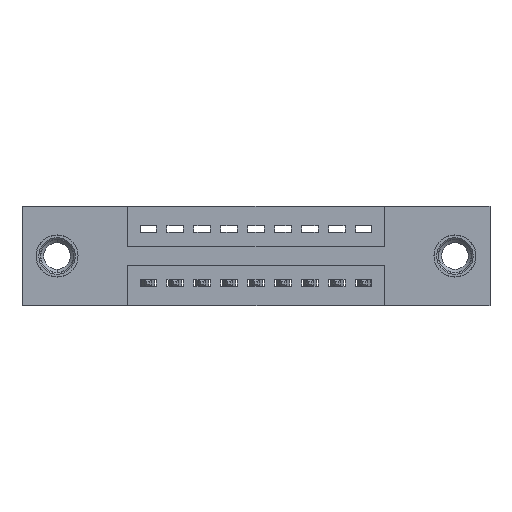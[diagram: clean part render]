
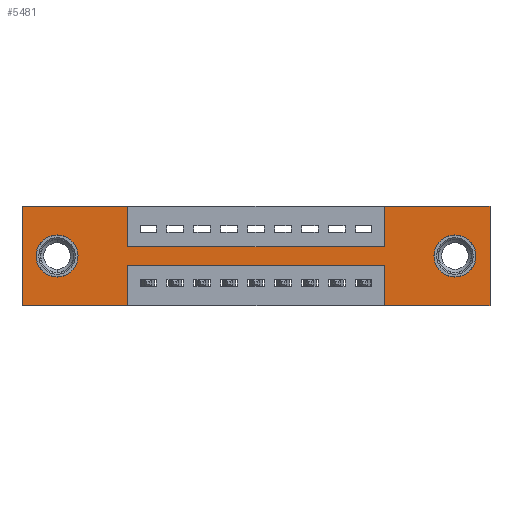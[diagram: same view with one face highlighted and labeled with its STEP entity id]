
A CAD part, front view. The second image highlights one B-rep face of the part: STEP entity #5481.
In plain terms, the highlighted planar face has unit normal (0, -1, 0).
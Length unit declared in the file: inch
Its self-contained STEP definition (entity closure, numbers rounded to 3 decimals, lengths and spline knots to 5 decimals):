
#288 = VECTOR ( 'NONE', #3596, 39.37008 ) ;
#349 = CARTESIAN_POINT ( 'NONE',  ( 1.605, 0., -0.185 ) ) ;
#390 = CIRCLE ( 'NONE', #5759, 0.078 ) ;
#465 = VERTEX_POINT ( 'NONE', #4016 ) ;
#560 = VERTEX_POINT ( 'NONE', #9679 ) ;
#705 = DIRECTION ( 'NONE',  ( 0., 0., -1. ) ) ;
#1059 = CARTESIAN_POINT ( 'NONE',  ( 0., 0., -0.37 ) ) ;
#1062 = CARTESIAN_POINT ( 'NONE',  ( 1.605, 0., -0.263 ) ) ;
#1087 = DIRECTION ( 'NONE',  ( 0., 1., 0. ) ) ;
#1147 = VECTOR ( 'NONE', #7812, 39.37008 ) ;
#1221 = VERTEX_POINT ( 'NONE', #8726 ) ;
#1239 = LINE ( 'NONE', #10455, #8635 ) ;
#1318 = FACE_BOUND ( 'NONE', #9086, .T. ) ;
#1320 = EDGE_CURVE ( 'NONE', #8238, #1763, #4493, .T. ) ;
#1367 = ORIENTED_EDGE ( 'NONE', *, *, #8337, .T. ) ;
#1380 = CARTESIAN_POINT ( 'NONE',  ( 1.3425, 0., -0.37 ) ) ;
#1414 = DIRECTION ( 'NONE',  ( 0., 0., -1. ) ) ;
#1483 = CARTESIAN_POINT ( 'NONE',  ( 0.3925, 0., 0. ) ) ;
#1697 = LINE ( 'NONE', #1380, #11542 ) ;
#1713 = CARTESIAN_POINT ( 'NONE',  ( 0.3925, 0., -0.22 ) ) ;
#1763 = VERTEX_POINT ( 'NONE', #12327 ) ;
#2135 = CARTESIAN_POINT ( 'NONE',  ( 0., 0., -0.37 ) ) ;
#2170 = CARTESIAN_POINT ( 'NONE',  ( 0., 0., -0.37 ) ) ;
#2295 = VERTEX_POINT ( 'NONE', #7875 ) ;
#2490 = EDGE_CURVE ( 'NONE', #6309, #8238, #1239, .T. ) ;
#2916 = LINE ( 'NONE', #3242, #7732 ) ;
#2983 = LINE ( 'NONE', #4534, #288 ) ;
#3011 = CARTESIAN_POINT ( 'NONE',  ( 0.3925, 0., -0.22 ) ) ;
#3021 = VERTEX_POINT ( 'NONE', #3043 ) ;
#3029 = VECTOR ( 'NONE', #6966, 39.37008 ) ;
#3043 = CARTESIAN_POINT ( 'NONE',  ( 0.13, 0., -0.263 ) ) ;
#3197 = VERTEX_POINT ( 'NONE', #1062 ) ;
#3242 = CARTESIAN_POINT ( 'NONE',  ( 0.3925, 0., -0.37 ) ) ;
#3250 = EDGE_CURVE ( 'NONE', #11455, #3021, #390, .T. ) ;
#3339 = CARTESIAN_POINT ( 'NONE',  ( 0.13, 0., -0.107 ) ) ;
#3596 = DIRECTION ( 'NONE',  ( 1., 0., 0. ) ) ;
#3654 = LINE ( 'NONE', #2135, #3029 ) ;
#3747 = LINE ( 'NONE', #6750, #8816 ) ;
#3754 = DIRECTION ( 'NONE',  ( 0., 1., 0. ) ) ;
#3777 = LINE ( 'NONE', #10648, #1147 ) ;
#3824 = DIRECTION ( 'NONE',  ( 0., 0., 1. ) ) ;
#3928 = VERTEX_POINT ( 'NONE', #6061 ) ;
#4016 = CARTESIAN_POINT ( 'NONE',  ( 0.3925, 0., -0.37 ) ) ;
#4255 = ORIENTED_EDGE ( 'NONE', *, *, #10203, .F. ) ;
#4257 = FACE_OUTER_BOUND ( 'NONE', #5708, .T. ) ;
#4493 = LINE ( 'NONE', #7409, #9558 ) ;
#4534 = CARTESIAN_POINT ( 'NONE',  ( 0.3925, 0., -0.15 ) ) ;
#4788 = ORIENTED_EDGE ( 'NONE', *, *, #9786, .T. ) ;
#5016 = DIRECTION ( 'NONE',  ( -1., 0., 0. ) ) ;
#5049 = CARTESIAN_POINT ( 'NONE',  ( 1.3425, 0., -0.22 ) ) ;
#5087 = EDGE_CURVE ( 'NONE', #465, #7644, #3654, .T. ) ;
#5103 = ORIENTED_EDGE ( 'NONE', *, *, #3250, .T. ) ;
#5397 = VECTOR ( 'NONE', #9446, 39.37008 ) ;
#5481 = ADVANCED_FACE ( 'NONE', ( #1318, #6528, #4257 ), #11275, .T. ) ;
#5586 = CIRCLE ( 'NONE', #11164, 0.078 ) ;
#5625 = DIRECTION ( 'NONE',  ( 0., 1., 0. ) ) ;
#5661 = CARTESIAN_POINT ( 'NONE',  ( 0., 0., -0.37 ) ) ;
#5683 = EDGE_CURVE ( 'NONE', #1763, #8829, #3777, .T. ) ;
#5708 = EDGE_LOOP ( 'NONE', ( #4255, #5980, #7627, #7581, #7399, #7213, #6256, #11023, #7398, #10986, #7903, #9835 ) ) ;
#5759 = AXIS2_PLACEMENT_3D ( 'NONE', #6928, #1087, #7863 ) ;
#5768 = ORIENTED_EDGE ( 'NONE', *, *, #7476, .T. ) ;
#5845 = CIRCLE ( 'NONE', #7458, 0.078 ) ;
#5980 = ORIENTED_EDGE ( 'NONE', *, *, #6327, .F. ) ;
#6061 = CARTESIAN_POINT ( 'NONE',  ( 1.3425, 0., -0.37 ) ) ;
#6256 = ORIENTED_EDGE ( 'NONE', *, *, #2490, .F. ) ;
#6309 = VERTEX_POINT ( 'NONE', #12356 ) ;
#6327 = EDGE_CURVE ( 'NONE', #9417, #6745, #9594, .T. ) ;
#6496 = LINE ( 'NONE', #1483, #8671 ) ;
#6528 = FACE_BOUND ( 'NONE', #11121, .T. ) ;
#6612 = DIRECTION ( 'NONE',  ( 0., -1., 0. ) ) ;
#6745 = VERTEX_POINT ( 'NONE', #1713 ) ;
#6750 = CARTESIAN_POINT ( 'NONE',  ( 0., 0., 0. ) ) ;
#6909 = CIRCLE ( 'NONE', #11816, 0.078 ) ;
#6928 = CARTESIAN_POINT ( 'NONE',  ( 0.13, 0., -0.185 ) ) ;
#6966 = DIRECTION ( 'NONE',  ( -1., 0., 0. ) ) ;
#7110 = DIRECTION ( 'NONE',  ( 0., 0., -1. ) ) ;
#7213 = ORIENTED_EDGE ( 'NONE', *, *, #1320, .F. ) ;
#7218 = DIRECTION ( 'NONE',  ( 0., 1., 0. ) ) ;
#7274 = EDGE_CURVE ( 'NONE', #9657, #560, #6496, .T. ) ;
#7348 = EDGE_CURVE ( 'NONE', #560, #6309, #2983, .T. ) ;
#7398 = ORIENTED_EDGE ( 'NONE', *, *, #7274, .F. ) ;
#7399 = ORIENTED_EDGE ( 'NONE', *, *, #5683, .F. ) ;
#7409 = CARTESIAN_POINT ( 'NONE',  ( 0., 0., 0. ) ) ;
#7458 = AXIS2_PLACEMENT_3D ( 'NONE', #11235, #5625, #12114 ) ;
#7476 = EDGE_CURVE ( 'NONE', #3197, #2295, #6909, .T. ) ;
#7543 = EDGE_CURVE ( 'NONE', #7644, #1221, #3747, .T. ) ;
#7581 = ORIENTED_EDGE ( 'NONE', *, *, #8830, .F. ) ;
#7627 = ORIENTED_EDGE ( 'NONE', *, *, #10281, .F. ) ;
#7644 = VERTEX_POINT ( 'NONE', #1059 ) ;
#7732 = VECTOR ( 'NONE', #7110, 39.37008 ) ;
#7812 = DIRECTION ( 'NONE',  ( 0., 0., -1. ) ) ;
#7863 = DIRECTION ( 'NONE',  ( 0., 0., 1. ) ) ;
#7875 = CARTESIAN_POINT ( 'NONE',  ( 1.605, 0., -0.107 ) ) ;
#7903 = ORIENTED_EDGE ( 'NONE', *, *, #7543, .F. ) ;
#8175 = LINE ( 'NONE', #12166, #5397 ) ;
#8238 = VERTEX_POINT ( 'NONE', #11754 ) ;
#8337 = EDGE_CURVE ( 'NONE', #2295, #3197, #5586, .T. ) ;
#8489 = VECTOR ( 'NONE', #10800, 39.37008 ) ;
#8514 = AXIS2_PLACEMENT_3D ( 'NONE', #5661, #6612, #705 ) ;
#8635 = VECTOR ( 'NONE', #10015, 39.37008 ) ;
#8671 = VECTOR ( 'NONE', #11081, 39.37008 ) ;
#8726 = CARTESIAN_POINT ( 'NONE',  ( 0., 0., 0. ) ) ;
#8816 = VECTOR ( 'NONE', #3824, 39.37008 ) ;
#8829 = VERTEX_POINT ( 'NONE', #11661 ) ;
#8830 = EDGE_CURVE ( 'NONE', #8829, #3928, #11004, .T. ) ;
#8981 = VECTOR ( 'NONE', #5016, 39.37008 ) ;
#9086 = EDGE_LOOP ( 'NONE', ( #1367, #5768 ) ) ;
#9324 = EDGE_CURVE ( 'NONE', #1221, #9657, #8175, .T. ) ;
#9417 = VERTEX_POINT ( 'NONE', #5049 ) ;
#9446 = DIRECTION ( 'NONE',  ( 1., 0., 0. ) ) ;
#9471 = CARTESIAN_POINT ( 'NONE',  ( 1.605, 0., -0.185 ) ) ;
#9558 = VECTOR ( 'NONE', #11094, 39.37008 ) ;
#9594 = LINE ( 'NONE', #3011, #8981 ) ;
#9657 = VERTEX_POINT ( 'NONE', #11042 ) ;
#9679 = CARTESIAN_POINT ( 'NONE',  ( 0.3925, 0., -0.15 ) ) ;
#9786 = EDGE_CURVE ( 'NONE', #3021, #11455, #5845, .T. ) ;
#9835 = ORIENTED_EDGE ( 'NONE', *, *, #5087, .F. ) ;
#10015 = DIRECTION ( 'NONE',  ( 0., 0., 1. ) ) ;
#10203 = EDGE_CURVE ( 'NONE', #6745, #465, #2916, .T. ) ;
#10281 = EDGE_CURVE ( 'NONE', #3928, #9417, #1697, .T. ) ;
#10433 = DIRECTION ( 'NONE',  ( 0., 0., -1. ) ) ;
#10455 = CARTESIAN_POINT ( 'NONE',  ( 1.3425, 0., 0. ) ) ;
#10648 = CARTESIAN_POINT ( 'NONE',  ( 1.735, 0., 0. ) ) ;
#10800 = DIRECTION ( 'NONE',  ( -1., 0., 0. ) ) ;
#10986 = ORIENTED_EDGE ( 'NONE', *, *, #9324, .F. ) ;
#11004 = LINE ( 'NONE', #2170, #8489 ) ;
#11023 = ORIENTED_EDGE ( 'NONE', *, *, #7348, .F. ) ;
#11042 = CARTESIAN_POINT ( 'NONE',  ( 0.3925, 0., 0. ) ) ;
#11081 = DIRECTION ( 'NONE',  ( 0., 0., -1. ) ) ;
#11094 = DIRECTION ( 'NONE',  ( 1., 0., 0. ) ) ;
#11121 = EDGE_LOOP ( 'NONE', ( #5103, #4788 ) ) ;
#11164 = AXIS2_PLACEMENT_3D ( 'NONE', #349, #7218, #1414 ) ;
#11235 = CARTESIAN_POINT ( 'NONE',  ( 0.13, 0., -0.185 ) ) ;
#11275 = PLANE ( 'NONE',  #8514 ) ;
#11455 = VERTEX_POINT ( 'NONE', #3339 ) ;
#11542 = VECTOR ( 'NONE', #11883, 39.37008 ) ;
#11661 = CARTESIAN_POINT ( 'NONE',  ( 1.735, 0., -0.37 ) ) ;
#11754 = CARTESIAN_POINT ( 'NONE',  ( 1.3425, 0., 0. ) ) ;
#11816 = AXIS2_PLACEMENT_3D ( 'NONE', #9471, #3754, #10433 ) ;
#11883 = DIRECTION ( 'NONE',  ( 0., 0., 1. ) ) ;
#12114 = DIRECTION ( 'NONE',  ( 0., 0., 1. ) ) ;
#12166 = CARTESIAN_POINT ( 'NONE',  ( 0., 0., 0. ) ) ;
#12327 = CARTESIAN_POINT ( 'NONE',  ( 1.735, 0., 0. ) ) ;
#12356 = CARTESIAN_POINT ( 'NONE',  ( 1.3425, 0., -0.15 ) ) ;
